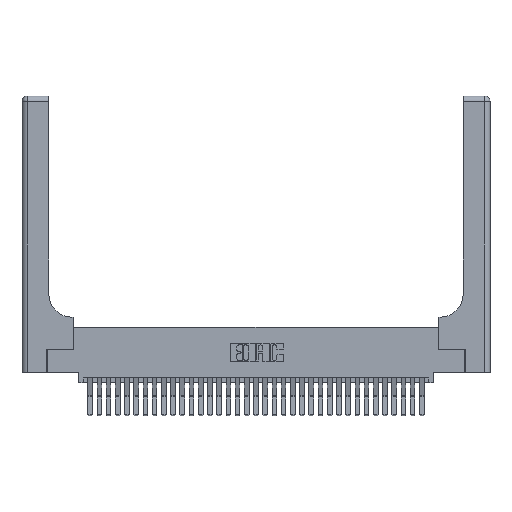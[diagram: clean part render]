
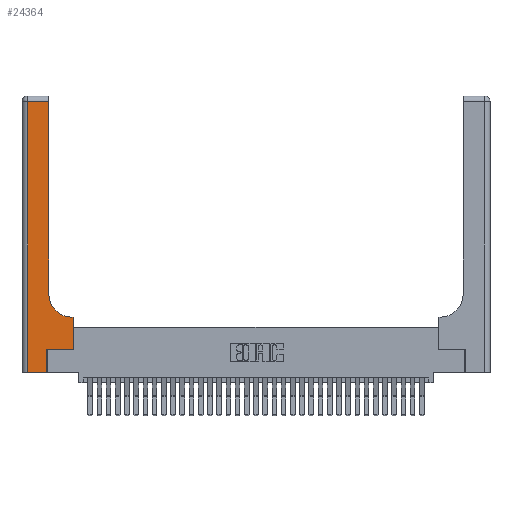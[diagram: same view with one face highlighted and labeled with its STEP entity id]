
A CAD part, top view. The second image highlights one B-rep face of the part: STEP entity #24364.
In plain terms, the highlighted planar face has unit normal (0, 0, 1).
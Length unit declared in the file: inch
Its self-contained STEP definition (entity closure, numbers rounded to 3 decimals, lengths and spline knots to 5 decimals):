
#425 = VECTOR ( 'NONE', #15198, 39.37008 ) ;
#490 = VECTOR ( 'NONE', #28088, 39.37008 ) ;
#1073 = CARTESIAN_POINT ( 'NONE',  ( 0.06, 0., 0.37 ) ) ;
#1861 = AXIS2_PLACEMENT_3D ( 'NONE', #25618, #9376, #28342 ) ;
#2083 = VERTEX_POINT ( 'NONE', #20621 ) ;
#2112 = DIRECTION ( 'NONE',  ( 0., 0., -1. ) ) ;
#2459 = CARTESIAN_POINT ( 'NONE',  ( 0.5585, 0.6, 0.37 ) ) ;
#2468 = CIRCLE ( 'NONE', #1861, 0.25 ) ;
#2988 = DIRECTION ( 'NONE',  ( 1., 0., 0. ) ) ;
#3268 = CARTESIAN_POINT ( 'NONE',  ( 0., 2.94, 0.37 ) ) ;
#3915 = DIRECTION ( 'NONE',  ( 0., 1., 0. ) ) ;
#4008 = VECTOR ( 'NONE', #2988, 39.37008 ) ;
#4687 = EDGE_CURVE ( 'NONE', #30003, #19180, #2468, .T. ) ;
#5066 = EDGE_CURVE ( 'NONE', #19180, #29998, #32975, .T. ) ;
#5342 = VECTOR ( 'NONE', #19577, 39.37008 ) ;
#5417 = CARTESIAN_POINT ( 'NONE',  ( 0.269, 0., 0.37 ) ) ;
#9376 = DIRECTION ( 'NONE',  ( 0., 0., -1. ) ) ;
#9728 = CARTESIAN_POINT ( 'NONE',  ( 0.269, 0.25, 0.37 ) ) ;
#10115 = EDGE_CURVE ( 'NONE', #21784, #34309, #15760, .T. ) ;
#11389 = VECTOR ( 'NONE', #33694, 39.37008 ) ;
#12022 = CARTESIAN_POINT ( 'NONE',  ( 0.2915, 0.6, 0.37 ) ) ;
#12054 = ORIENTED_EDGE ( 'NONE', *, *, #5066, .T. ) ;
#12572 = LINE ( 'NONE', #3268, #5342 ) ;
#13499 = EDGE_CURVE ( 'NONE', #2083, #17656, #29165, .T. ) ;
#14222 = EDGE_CURVE ( 'NONE', #26140, #2083, #21524, .T. ) ;
#14390 = DIRECTION ( 'NONE',  ( 1., 0., 0. ) ) ;
#14896 = CARTESIAN_POINT ( 'NONE',  ( 0.06, 2.94, 0.37 ) ) ;
#14962 = ORIENTED_EDGE ( 'NONE', *, *, #26433, .T. ) ;
#15198 = DIRECTION ( 'NONE',  ( 0., -1., 0. ) ) ;
#15676 = CARTESIAN_POINT ( 'NONE',  ( 0., 3., 0.37 ) ) ;
#15760 = LINE ( 'NONE', #25964, #425 ) ;
#15764 = EDGE_CURVE ( 'NONE', #34309, #24527, #24825, .T. ) ;
#16565 = CARTESIAN_POINT ( 'NONE',  ( 0., 0., 0.37 ) ) ;
#16633 = CARTESIAN_POINT ( 'NONE',  ( 0.2915, 2.94, 0.37 ) ) ;
#17129 = CARTESIAN_POINT ( 'NONE',  ( 0.269, 0.25, 0.37 ) ) ;
#17235 = EDGE_CURVE ( 'NONE', #24527, #26140, #22201, .T. ) ;
#17656 = VERTEX_POINT ( 'NONE', #2459 ) ;
#18721 = ORIENTED_EDGE ( 'NONE', *, *, #4687, .T. ) ;
#19180 = VERTEX_POINT ( 'NONE', #25743 ) ;
#19577 = DIRECTION ( 'NONE',  ( -1., 0., 0. ) ) ;
#19842 = ORIENTED_EDGE ( 'NONE', *, *, #17235, .T. ) ;
#20480 = ORIENTED_EDGE ( 'NONE', *, *, #25346, .T. ) ;
#20621 = CARTESIAN_POINT ( 'NONE',  ( 0.5585, 0.25, 0.37 ) ) ;
#21145 = DIRECTION ( 'NONE',  ( -1., 0., 0. ) ) ;
#21524 = LINE ( 'NONE', #17129, #35024 ) ;
#21624 = ORIENTED_EDGE ( 'NONE', *, *, #15764, .T. ) ;
#21784 = VERTEX_POINT ( 'NONE', #14896 ) ;
#21861 = CARTESIAN_POINT ( 'NONE',  ( 0.5415, 0.6, 0.37 ) ) ;
#21990 = VECTOR ( 'NONE', #28951, 39.37008 ) ;
#22201 = LINE ( 'NONE', #25388, #490 ) ;
#23570 = EDGE_LOOP ( 'NONE', ( #12054, #14962, #28798, #21624, #19842, #23946, #29617, #20480, #18721 ) ) ;
#23946 = ORIENTED_EDGE ( 'NONE', *, *, #14222, .T. ) ;
#24364 = ADVANCED_FACE ( 'NONE', ( #33061 ), #31873, .F. ) ;
#24527 = VERTEX_POINT ( 'NONE', #5417 ) ;
#24825 = LINE ( 'NONE', #16565, #4008 ) ;
#25346 = EDGE_CURVE ( 'NONE', #17656, #30003, #25826, .T. ) ;
#25388 = CARTESIAN_POINT ( 'NONE',  ( 0.269, 0., 0.37 ) ) ;
#25618 = CARTESIAN_POINT ( 'NONE',  ( 0.5415, 0.85, 0.37 ) ) ;
#25743 = CARTESIAN_POINT ( 'NONE',  ( 0.2915, 0.85, 0.37 ) ) ;
#25803 = VECTOR ( 'NONE', #3915, 39.37008 ) ;
#25826 = LINE ( 'NONE', #12022, #11389 ) ;
#25964 = CARTESIAN_POINT ( 'NONE',  ( 0.06, 3., 0.37 ) ) ;
#26140 = VERTEX_POINT ( 'NONE', #9728 ) ;
#26433 = EDGE_CURVE ( 'NONE', #29998, #21784, #12572, .T. ) ;
#28088 = DIRECTION ( 'NONE',  ( 0., 1., 0. ) ) ;
#28342 = DIRECTION ( 'NONE',  ( 1., 0., 0. ) ) ;
#28798 = ORIENTED_EDGE ( 'NONE', *, *, #10115, .T. ) ;
#28951 = DIRECTION ( 'NONE',  ( 0., 1., 0. ) ) ;
#29165 = LINE ( 'NONE', #34278, #21990 ) ;
#29617 = ORIENTED_EDGE ( 'NONE', *, *, #13499, .T. ) ;
#29998 = VERTEX_POINT ( 'NONE', #16633 ) ;
#30003 = VERTEX_POINT ( 'NONE', #21861 ) ;
#30665 = AXIS2_PLACEMENT_3D ( 'NONE', #15676, #2112, #21145 ) ;
#31873 = PLANE ( 'NONE',  #30665 ) ;
#32975 = LINE ( 'NONE', #33674, #25803 ) ;
#33061 = FACE_OUTER_BOUND ( 'NONE', #23570, .T. ) ;
#33674 = CARTESIAN_POINT ( 'NONE',  ( 0.2915, 3., 0.37 ) ) ;
#33694 = DIRECTION ( 'NONE',  ( -1., 0., 0. ) ) ;
#34278 = CARTESIAN_POINT ( 'NONE',  ( 0.5585, 0.25, 0.37 ) ) ;
#34309 = VERTEX_POINT ( 'NONE', #1073 ) ;
#35024 = VECTOR ( 'NONE', #14390, 39.37008 ) ;
